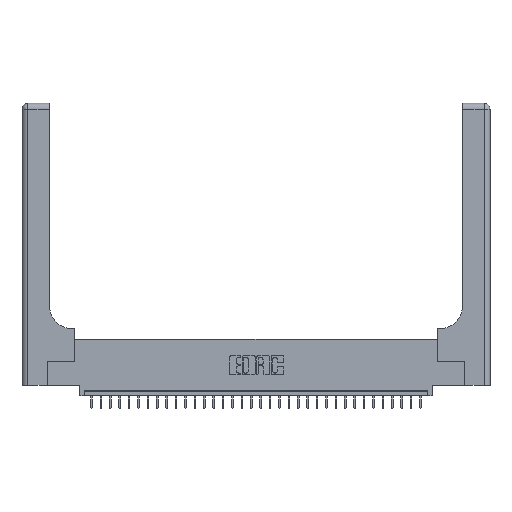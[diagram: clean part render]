
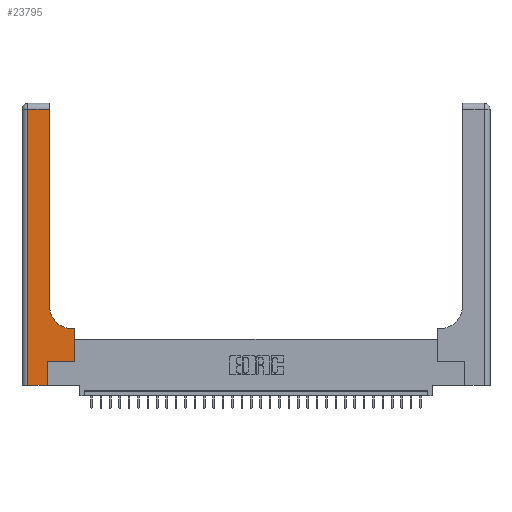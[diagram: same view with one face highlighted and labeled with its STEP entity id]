
A CAD part, top view. The second image highlights one B-rep face of the part: STEP entity #23795.
In plain terms, the highlighted planar face has unit normal (0, 0, 1).
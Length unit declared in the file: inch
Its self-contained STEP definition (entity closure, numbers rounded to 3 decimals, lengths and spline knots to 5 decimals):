
#495 = LINE ( 'NONE', #25957, #22671 ) ;
#1081 = CARTESIAN_POINT ( 'NONE',  ( 0.269, 0.25, 0.37 ) ) ;
#1132 = DIRECTION ( 'NONE',  ( 0., 0., -1. ) ) ;
#1824 = LINE ( 'NONE', #27941, #27629 ) ;
#3443 = CARTESIAN_POINT ( 'NONE',  ( 0.5415, 0.6, 0.37 ) ) ;
#4032 = EDGE_LOOP ( 'NONE', ( #24116, #19185, #30867, #6900, #30068, #6494, #20392, #6623, #4851 ) ) ;
#4299 = VECTOR ( 'NONE', #19438, 39.37008 ) ;
#4539 = VECTOR ( 'NONE', #31419, 39.37008 ) ;
#4829 = LINE ( 'NONE', #27915, #30725 ) ;
#4851 = ORIENTED_EDGE ( 'NONE', *, *, #20781, .T. ) ;
#5372 = VECTOR ( 'NONE', #9507, 39.37008 ) ;
#5569 = CARTESIAN_POINT ( 'NONE',  ( 0.5415, 0.85, 0.37 ) ) ;
#5706 = LINE ( 'NONE', #18485, #4299 ) ;
#5988 = CARTESIAN_POINT ( 'NONE',  ( 0.2915, 3., 0.37 ) ) ;
#6189 = CARTESIAN_POINT ( 'NONE',  ( 0., 3., 0.37 ) ) ;
#6407 = CARTESIAN_POINT ( 'NONE',  ( 0.2915, 0.85, 0.37 ) ) ;
#6494 = ORIENTED_EDGE ( 'NONE', *, *, #13036, .T. ) ;
#6623 = ORIENTED_EDGE ( 'NONE', *, *, #27892, .T. ) ;
#6900 = ORIENTED_EDGE ( 'NONE', *, *, #13947, .T. ) ;
#7375 = EDGE_CURVE ( 'NONE', #18406, #13597, #1824, .T. ) ;
#8256 = FACE_OUTER_BOUND ( 'NONE', #4032, .T. ) ;
#8599 = VECTOR ( 'NONE', #18750, 39.37008 ) ;
#8670 = EDGE_CURVE ( 'NONE', #18280, #18406, #28898, .T. ) ;
#9115 = CARTESIAN_POINT ( 'NONE',  ( 0.06, 2.94, 0.37 ) ) ;
#9507 = DIRECTION ( 'NONE',  ( -1., 0., 0. ) ) ;
#10058 = DIRECTION ( 'NONE',  ( 0., 1., 0. ) ) ;
#11050 = AXIS2_PLACEMENT_3D ( 'NONE', #5569, #17682, #20547 ) ;
#11395 = EDGE_CURVE ( 'NONE', #27026, #22077, #20497, .T. ) ;
#13036 = EDGE_CURVE ( 'NONE', #22077, #26727, #31906, .T. ) ;
#13597 = VERTEX_POINT ( 'NONE', #9115 ) ;
#13947 = EDGE_CURVE ( 'NONE', #17123, #27026, #4829, .T. ) ;
#14508 = VECTOR ( 'NONE', #10058, 39.37008 ) ;
#15165 = CARTESIAN_POINT ( 'NONE',  ( 0.2915, 2.94, 0.37 ) ) ;
#16437 = CIRCLE ( 'NONE', #11050, 0.25 ) ;
#17123 = VERTEX_POINT ( 'NONE', #25431 ) ;
#17682 = DIRECTION ( 'NONE',  ( 0., 0., -1. ) ) ;
#18280 = VERTEX_POINT ( 'NONE', #6407 ) ;
#18406 = VERTEX_POINT ( 'NONE', #15165 ) ;
#18485 = CARTESIAN_POINT ( 'NONE',  ( 0.06, 3., 0.37 ) ) ;
#18523 = PLANE ( 'NONE',  #32640 ) ;
#18750 = DIRECTION ( 'NONE',  ( 1., 0., 0. ) ) ;
#18843 = CARTESIAN_POINT ( 'NONE',  ( 0.5585, 0.6, 0.37 ) ) ;
#19185 = ORIENTED_EDGE ( 'NONE', *, *, #7375, .T. ) ;
#19438 = DIRECTION ( 'NONE',  ( 0., -1., 0. ) ) ;
#20110 = VERTEX_POINT ( 'NONE', #3443 ) ;
#20392 = ORIENTED_EDGE ( 'NONE', *, *, #31900, .T. ) ;
#20497 = LINE ( 'NONE', #22859, #14508 ) ;
#20547 = DIRECTION ( 'NONE',  ( 1., 0., 0. ) ) ;
#20781 = EDGE_CURVE ( 'NONE', #20110, #18280, #16437, .T. ) ;
#21951 = VERTEX_POINT ( 'NONE', #18843 ) ;
#22077 = VERTEX_POINT ( 'NONE', #22393 ) ;
#22393 = CARTESIAN_POINT ( 'NONE',  ( 0.269, 0.25, 0.37 ) ) ;
#22629 = CARTESIAN_POINT ( 'NONE',  ( 0.2915, 0.6, 0.37 ) ) ;
#22671 = VECTOR ( 'NONE', #23733, 39.37008 ) ;
#22753 = CARTESIAN_POINT ( 'NONE',  ( 0.269, 0., 0.37 ) ) ;
#22859 = CARTESIAN_POINT ( 'NONE',  ( 0.269, 0., 0.37 ) ) ;
#23733 = DIRECTION ( 'NONE',  ( 0., 1., 0. ) ) ;
#23795 = ADVANCED_FACE ( 'NONE', ( #8256 ), #18523, .F. ) ;
#24116 = ORIENTED_EDGE ( 'NONE', *, *, #8670, .T. ) ;
#24190 = DIRECTION ( 'NONE',  ( -1., 0., 0. ) ) ;
#25339 = LINE ( 'NONE', #22629, #5372 ) ;
#25431 = CARTESIAN_POINT ( 'NONE',  ( 0.06, 0., 0.37 ) ) ;
#25957 = CARTESIAN_POINT ( 'NONE',  ( 0.5585, 0.25, 0.37 ) ) ;
#26727 = VERTEX_POINT ( 'NONE', #31196 ) ;
#27026 = VERTEX_POINT ( 'NONE', #22753 ) ;
#27629 = VECTOR ( 'NONE', #32479, 39.37008 ) ;
#27714 = EDGE_CURVE ( 'NONE', #13597, #17123, #5706, .T. ) ;
#27892 = EDGE_CURVE ( 'NONE', #21951, #20110, #25339, .T. ) ;
#27915 = CARTESIAN_POINT ( 'NONE',  ( 0., 0., 0.37 ) ) ;
#27941 = CARTESIAN_POINT ( 'NONE',  ( 0., 2.94, 0.37 ) ) ;
#28898 = LINE ( 'NONE', #5988, #4539 ) ;
#30068 = ORIENTED_EDGE ( 'NONE', *, *, #11395, .T. ) ;
#30725 = VECTOR ( 'NONE', #32613, 39.37008 ) ;
#30867 = ORIENTED_EDGE ( 'NONE', *, *, #27714, .T. ) ;
#31196 = CARTESIAN_POINT ( 'NONE',  ( 0.5585, 0.25, 0.37 ) ) ;
#31419 = DIRECTION ( 'NONE',  ( 0., 1., 0. ) ) ;
#31900 = EDGE_CURVE ( 'NONE', #26727, #21951, #495, .T. ) ;
#31906 = LINE ( 'NONE', #1081, #8599 ) ;
#32479 = DIRECTION ( 'NONE',  ( -1., 0., 0. ) ) ;
#32613 = DIRECTION ( 'NONE',  ( 1., 0., 0. ) ) ;
#32640 = AXIS2_PLACEMENT_3D ( 'NONE', #6189, #1132, #24190 ) ;
